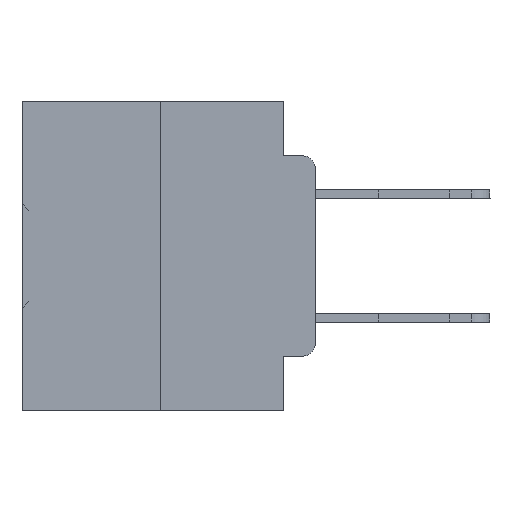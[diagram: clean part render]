
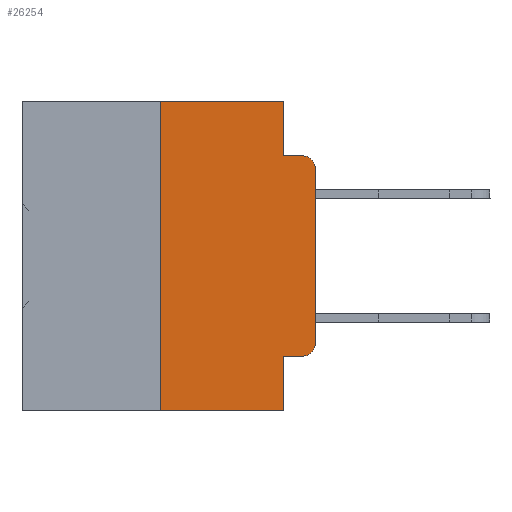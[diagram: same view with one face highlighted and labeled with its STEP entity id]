
A CAD part, left-side view. The second image highlights one B-rep face of the part: STEP entity #26254.
In plain terms, the highlighted planar face has unit normal (-1, 0, 0).
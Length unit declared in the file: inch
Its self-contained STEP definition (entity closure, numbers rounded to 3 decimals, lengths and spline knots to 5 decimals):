
#629 = EDGE_CURVE ( 'NONE', #39630, #19291, #30210, .T. ) ;
#704 = AXIS2_PLACEMENT_3D ( 'NONE', #16661, #38190, #19801 ) ;
#1038 = LINE ( 'NONE', #36619, #33039 ) ;
#1057 = DIRECTION ( 'NONE',  ( 0., -1., 0. ) ) ;
#2379 = DIRECTION ( 'NONE',  ( 0., 0., 1. ) ) ;
#2728 = EDGE_CURVE ( 'NONE', #13345, #31652, #21907, .T. ) ;
#2886 = DIRECTION ( 'NONE',  ( 0., -1., 0. ) ) ;
#2979 = CARTESIAN_POINT ( 'NONE',  ( 0., 0.051, -0.0885 ) ) ;
#3280 = CARTESIAN_POINT ( 'NONE',  ( 0., 0.02, -0.3915 ) ) ;
#3707 = ORIENTED_EDGE ( 'NONE', *, *, #11038, .F. ) ;
#4497 = VECTOR ( 'NONE', #2886, 39.37008 ) ;
#5061 = CARTESIAN_POINT ( 'NONE',  ( 0., 0.473, 0. ) ) ;
#5360 = EDGE_CURVE ( 'NONE', #13345, #19291, #22594, .T. ) ;
#5418 = VERTEX_POINT ( 'NONE', #40005 ) ;
#6107 = DIRECTION ( 'NONE',  ( 0., 0., 1. ) ) ;
#6378 = CARTESIAN_POINT ( 'NONE',  ( 0., 0.051, 0. ) ) ;
#6402 = DIRECTION ( 'NONE',  ( 0., 0., -1. ) ) ;
#6904 = EDGE_CURVE ( 'NONE', #34263, #32261, #1038, .T. ) ;
#8166 = DIRECTION ( 'NONE',  ( 0., 0., -1. ) ) ;
#10271 = CARTESIAN_POINT ( 'NONE',  ( 0., 0.473, 0. ) ) ;
#11038 = EDGE_CURVE ( 'NONE', #32261, #25914, #12781, .T. ) ;
#12099 = CIRCLE ( 'NONE', #704, 0.02 ) ;
#12781 = LINE ( 'NONE', #18378, #4497 ) ;
#13001 = AXIS2_PLACEMENT_3D ( 'NONE', #3280, #25042, #6402 ) ;
#13151 = EDGE_CURVE ( 'NONE', #37317, #25914, #12099, .T. ) ;
#13345 = VERTEX_POINT ( 'NONE', #29910 ) ;
#14289 = PLANE ( 'NONE',  #25113 ) ;
#14294 = VECTOR ( 'NONE', #30681, 39.37008 ) ;
#15296 = VECTOR ( 'NONE', #1057, 39.37008 ) ;
#15519 = EDGE_CURVE ( 'NONE', #31652, #34263, #16300, .T. ) ;
#15764 = CARTESIAN_POINT ( 'NONE',  ( 0., 0.051, -0.4115 ) ) ;
#16300 = LINE ( 'NONE', #10271, #15296 ) ;
#16661 = CARTESIAN_POINT ( 'NONE',  ( 0., 0.02, -0.1085 ) ) ;
#17306 = EDGE_CURVE ( 'NONE', #5418, #37317, #17643, .T. ) ;
#17643 = LINE ( 'NONE', #24736, #34985 ) ;
#18378 = CARTESIAN_POINT ( 'NONE',  ( 0., 0.051, -0.0885 ) ) ;
#18850 = ORIENTED_EDGE ( 'NONE', *, *, #6904, .F. ) ;
#19291 = VERTEX_POINT ( 'NONE', #32529 ) ;
#19801 = DIRECTION ( 'NONE',  ( 0., 0., -1. ) ) ;
#20800 = ORIENTED_EDGE ( 'NONE', *, *, #15519, .F. ) ;
#21197 = ORIENTED_EDGE ( 'NONE', *, *, #13151, .T. ) ;
#21294 = EDGE_LOOP ( 'NONE', ( #29721, #21197, #3707, #18850, #20800, #21784, #34147, #35700, #35880, #35957 ) ) ;
#21370 = CARTESIAN_POINT ( 'NONE',  ( 0., 0.473, -0.5 ) ) ;
#21784 = ORIENTED_EDGE ( 'NONE', *, *, #2728, .F. ) ;
#21798 = CARTESIAN_POINT ( 'NONE',  ( 0., 0.25, 0. ) ) ;
#21907 = LINE ( 'NONE', #33247, #28152 ) ;
#22276 = DIRECTION ( 'NONE',  ( 0., 0., -1. ) ) ;
#22594 = LINE ( 'NONE', #21370, #14294 ) ;
#24606 = DIRECTION ( 'NONE',  ( 0., 0., -1. ) ) ;
#24736 = CARTESIAN_POINT ( 'NONE',  ( 0., 0., 0. ) ) ;
#25042 = DIRECTION ( 'NONE',  ( -1., 0., 0. ) ) ;
#25113 = AXIS2_PLACEMENT_3D ( 'NONE', #5061, #26772, #8166 ) ;
#25505 = CARTESIAN_POINT ( 'NONE',  ( 0., 0., -0.1085 ) ) ;
#25914 = VERTEX_POINT ( 'NONE', #34294 ) ;
#26254 = ADVANCED_FACE ( 'NONE', ( #33967 ), #14289, .F. ) ;
#26772 = DIRECTION ( 'NONE',  ( 1., 0., 0. ) ) ;
#27577 = CIRCLE ( 'NONE', #13001, 0.02 ) ;
#28152 = VECTOR ( 'NONE', #2379, 39.37008 ) ;
#28538 = CARTESIAN_POINT ( 'NONE',  ( 0., 0.02, -0.4115 ) ) ;
#29721 = ORIENTED_EDGE ( 'NONE', *, *, #17306, .T. ) ;
#29910 = CARTESIAN_POINT ( 'NONE',  ( 0., 0.25, -0.5 ) ) ;
#30210 = LINE ( 'NONE', #6378, #38320 ) ;
#30681 = DIRECTION ( 'NONE',  ( 0., -1., 0. ) ) ;
#31472 = DIRECTION ( 'NONE',  ( 0., -1., 0. ) ) ;
#31652 = VERTEX_POINT ( 'NONE', #21798 ) ;
#32122 = VECTOR ( 'NONE', #31472, 39.37008 ) ;
#32261 = VERTEX_POINT ( 'NONE', #2979 ) ;
#32529 = CARTESIAN_POINT ( 'NONE',  ( 0., 0.051, -0.5 ) ) ;
#32583 = EDGE_CURVE ( 'NONE', #39819, #5418, #27577, .T. ) ;
#33039 = VECTOR ( 'NONE', #24606, 39.37008 ) ;
#33247 = CARTESIAN_POINT ( 'NONE',  ( 0., 0.25, 0. ) ) ;
#33967 = FACE_OUTER_BOUND ( 'NONE', #21294, .T. ) ;
#34002 = LINE ( 'NONE', #15764, #32122 ) ;
#34147 = ORIENTED_EDGE ( 'NONE', *, *, #5360, .T. ) ;
#34263 = VERTEX_POINT ( 'NONE', #39496 ) ;
#34294 = CARTESIAN_POINT ( 'NONE',  ( 0., 0.02, -0.0885 ) ) ;
#34985 = VECTOR ( 'NONE', #6107, 39.37008 ) ;
#35700 = ORIENTED_EDGE ( 'NONE', *, *, #629, .F. ) ;
#35880 = ORIENTED_EDGE ( 'NONE', *, *, #36631, .T. ) ;
#35957 = ORIENTED_EDGE ( 'NONE', *, *, #32583, .T. ) ;
#36619 = CARTESIAN_POINT ( 'NONE',  ( 0., 0.051, 0. ) ) ;
#36631 = EDGE_CURVE ( 'NONE', #39630, #39819, #34002, .T. ) ;
#37317 = VERTEX_POINT ( 'NONE', #25505 ) ;
#38190 = DIRECTION ( 'NONE',  ( -1., 0., 0. ) ) ;
#38320 = VECTOR ( 'NONE', #22276, 39.37008 ) ;
#39496 = CARTESIAN_POINT ( 'NONE',  ( 0., 0.051, 0. ) ) ;
#39630 = VERTEX_POINT ( 'NONE', #39914 ) ;
#39819 = VERTEX_POINT ( 'NONE', #28538 ) ;
#39914 = CARTESIAN_POINT ( 'NONE',  ( 0., 0.051, -0.4115 ) ) ;
#40005 = CARTESIAN_POINT ( 'NONE',  ( 0., 0., -0.3915 ) ) ;
